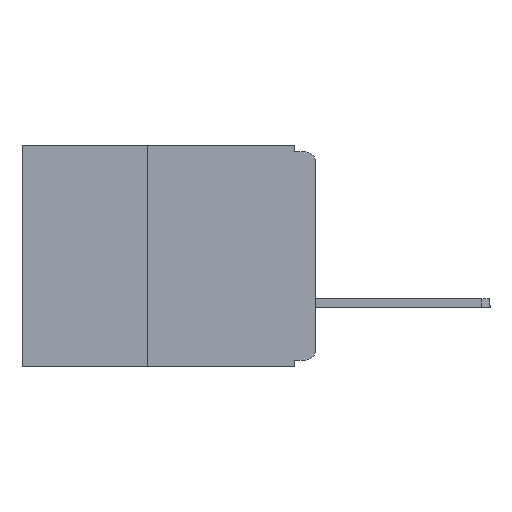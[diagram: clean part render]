
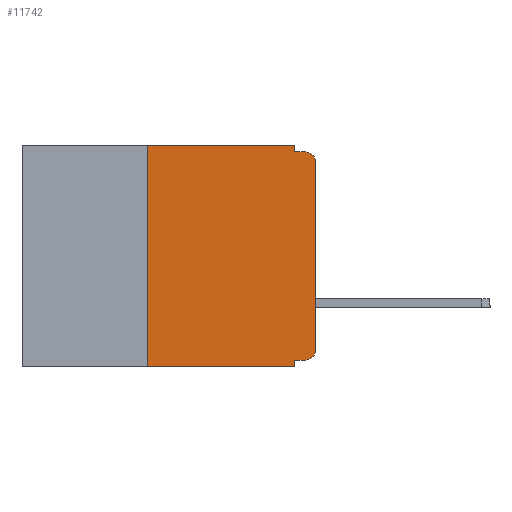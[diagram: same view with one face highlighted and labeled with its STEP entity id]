
A CAD part, left-side view. The second image highlights one B-rep face of the part: STEP entity #11742.
In plain terms, the highlighted planar face has unit normal (-1, 0, 0).
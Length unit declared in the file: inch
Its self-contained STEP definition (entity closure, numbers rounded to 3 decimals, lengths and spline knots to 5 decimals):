
#401 = VECTOR ( 'NONE', #986, 39.37008 ) ;
#986 = DIRECTION ( 'NONE',  ( 0., 0., -1. ) ) ;
#1024 = ORIENTED_EDGE ( 'NONE', *, *, #12701, .T. ) ;
#1235 = VECTOR ( 'NONE', #1379, 39.37008 ) ;
#1379 = DIRECTION ( 'NONE',  ( 0., 0., -1. ) ) ;
#2551 = CARTESIAN_POINT ( 'NONE',  ( 0., 0., 0. ) ) ;
#3076 = ORIENTED_EDGE ( 'NONE', *, *, #12910, .T. ) ;
#3196 = CARTESIAN_POINT ( 'NONE',  ( 0., 0.015, -0.01 ) ) ;
#4027 = CARTESIAN_POINT ( 'NONE',  ( 0., 0.031, 0. ) ) ;
#5079 = VERTEX_POINT ( 'NONE', #15566 ) ;
#5265 = DIRECTION ( 'NONE',  ( 0., 1., 0. ) ) ;
#5823 = CARTESIAN_POINT ( 'NONE',  ( 0., 0.015, -0.025 ) ) ;
#6067 = FACE_OUTER_BOUND ( 'NONE', #9101, .T. ) ;
#6632 = ORIENTED_EDGE ( 'NONE', *, *, #30577, .T. ) ;
#7243 = DIRECTION ( 'NONE',  ( 1., 0., 0. ) ) ;
#7306 = VECTOR ( 'NONE', #23241, 39.37008 ) ;
#7570 = LINE ( 'NONE', #22437, #401 ) ;
#7643 = LINE ( 'NONE', #20542, #1235 ) ;
#7730 = LINE ( 'NONE', #17663, #18917 ) ;
#8152 = VERTEX_POINT ( 'NONE', #3196 ) ;
#8253 = DIRECTION ( 'NONE',  ( 0., 0., -1. ) ) ;
#8796 = ORIENTED_EDGE ( 'NONE', *, *, #27768, .F. ) ;
#8866 = EDGE_CURVE ( 'NONE', #27207, #10778, #7730, .T. ) ;
#9101 = EDGE_LOOP ( 'NONE', ( #3076, #6632, #30578, #22531, #25562, #29281, #1024, #19434, #8796, #22435 ) ) ;
#10121 = EDGE_CURVE ( 'NONE', #14216, #14413, #7643, .T. ) ;
#10494 = CARTESIAN_POINT ( 'NONE',  ( 0., 0., -0.025 ) ) ;
#10608 = EDGE_CURVE ( 'NONE', #18813, #25567, #14392, .T. ) ;
#10676 = EDGE_CURVE ( 'NONE', #5079, #8152, #12160, .T. ) ;
#10778 = VERTEX_POINT ( 'NONE', #17826 ) ;
#10926 = VERTEX_POINT ( 'NONE', #4027 ) ;
#11742 = ADVANCED_FACE ( 'NONE', ( #6067 ), #28476, .F. ) ;
#12160 = LINE ( 'NONE', #24569, #23311 ) ;
#12447 = DIRECTION ( 'NONE',  ( -1., 0., 0. ) ) ;
#12701 = EDGE_CURVE ( 'NONE', #27207, #14413, #13673, .T. ) ;
#12910 = EDGE_CURVE ( 'NONE', #25567, #19180, #13283, .T. ) ;
#13148 = LINE ( 'NONE', #26665, #24275 ) ;
#13283 = LINE ( 'NONE', #2551, #20386 ) ;
#13673 = LINE ( 'NONE', #20774, #7306 ) ;
#13887 = CARTESIAN_POINT ( 'NONE',  ( 0., 0.031, -0.32 ) ) ;
#14216 = VERTEX_POINT ( 'NONE', #13887 ) ;
#14392 = CIRCLE ( 'NONE', #14612, 0.015 ) ;
#14413 = VERTEX_POINT ( 'NONE', #21788 ) ;
#14612 = AXIS2_PLACEMENT_3D ( 'NONE', #26604, #12447, #28941 ) ;
#15290 = CIRCLE ( 'NONE', #26579, 0.015 ) ;
#15566 = CARTESIAN_POINT ( 'NONE',  ( 0., 0.031, -0.01 ) ) ;
#16864 = DIRECTION ( 'NONE',  ( 0., 0., 1. ) ) ;
#17171 = DIRECTION ( 'NONE',  ( 0., -1., 0. ) ) ;
#17406 = DIRECTION ( 'NONE',  ( 0., -1., 0. ) ) ;
#17663 = CARTESIAN_POINT ( 'NONE',  ( 0., 0.25, -0.33 ) ) ;
#17826 = CARTESIAN_POINT ( 'NONE',  ( 0., 0.25, 0. ) ) ;
#18813 = VERTEX_POINT ( 'NONE', #21054 ) ;
#18917 = VECTOR ( 'NONE', #24814, 39.37008 ) ;
#19180 = VERTEX_POINT ( 'NONE', #10494 ) ;
#19434 = ORIENTED_EDGE ( 'NONE', *, *, #10121, .F. ) ;
#19484 = CARTESIAN_POINT ( 'NONE',  ( 0., 0.437, 0. ) ) ;
#20350 = EDGE_CURVE ( 'NONE', #10778, #10926, #27550, .T. ) ;
#20386 = VECTOR ( 'NONE', #16864, 39.37008 ) ;
#20542 = CARTESIAN_POINT ( 'NONE',  ( 0., 0.031, -0.33 ) ) ;
#20594 = VECTOR ( 'NONE', #17171, 39.37008 ) ;
#20774 = CARTESIAN_POINT ( 'NONE',  ( 0., 0.437, -0.33 ) ) ;
#21054 = CARTESIAN_POINT ( 'NONE',  ( 0., 0.015, -0.32 ) ) ;
#21546 = CARTESIAN_POINT ( 'NONE',  ( 0., 0.437, 0. ) ) ;
#21788 = CARTESIAN_POINT ( 'NONE',  ( 0., 0.031, -0.33 ) ) ;
#21825 = AXIS2_PLACEMENT_3D ( 'NONE', #21546, #7243, #23899 ) ;
#22435 = ORIENTED_EDGE ( 'NONE', *, *, #10608, .T. ) ;
#22437 = CARTESIAN_POINT ( 'NONE',  ( 0., 0.031, 0. ) ) ;
#22531 = ORIENTED_EDGE ( 'NONE', *, *, #27276, .F. ) ;
#22537 = DIRECTION ( 'NONE',  ( -1., 0., 0. ) ) ;
#23241 = DIRECTION ( 'NONE',  ( 0., -1., 0. ) ) ;
#23311 = VECTOR ( 'NONE', #17406, 39.37008 ) ;
#23899 = DIRECTION ( 'NONE',  ( 0., 0., -1. ) ) ;
#24275 = VECTOR ( 'NONE', #5265, 39.37008 ) ;
#24569 = CARTESIAN_POINT ( 'NONE',  ( 0., 0., -0.01 ) ) ;
#24574 = CARTESIAN_POINT ( 'NONE',  ( 0., 0.25, -0.33 ) ) ;
#24814 = DIRECTION ( 'NONE',  ( 0., 0., 1. ) ) ;
#25562 = ORIENTED_EDGE ( 'NONE', *, *, #20350, .F. ) ;
#25567 = VERTEX_POINT ( 'NONE', #26181 ) ;
#26181 = CARTESIAN_POINT ( 'NONE',  ( 0., 0., -0.305 ) ) ;
#26579 = AXIS2_PLACEMENT_3D ( 'NONE', #5823, #22537, #8253 ) ;
#26604 = CARTESIAN_POINT ( 'NONE',  ( 0., 0.015, -0.305 ) ) ;
#26665 = CARTESIAN_POINT ( 'NONE',  ( 0., 0., -0.32 ) ) ;
#27207 = VERTEX_POINT ( 'NONE', #24574 ) ;
#27276 = EDGE_CURVE ( 'NONE', #10926, #5079, #7570, .T. ) ;
#27550 = LINE ( 'NONE', #19484, #20594 ) ;
#27768 = EDGE_CURVE ( 'NONE', #18813, #14216, #13148, .T. ) ;
#28476 = PLANE ( 'NONE',  #21825 ) ;
#28941 = DIRECTION ( 'NONE',  ( 0., 0., -1. ) ) ;
#29281 = ORIENTED_EDGE ( 'NONE', *, *, #8866, .F. ) ;
#30577 = EDGE_CURVE ( 'NONE', #19180, #8152, #15290, .T. ) ;
#30578 = ORIENTED_EDGE ( 'NONE', *, *, #10676, .F. ) ;
